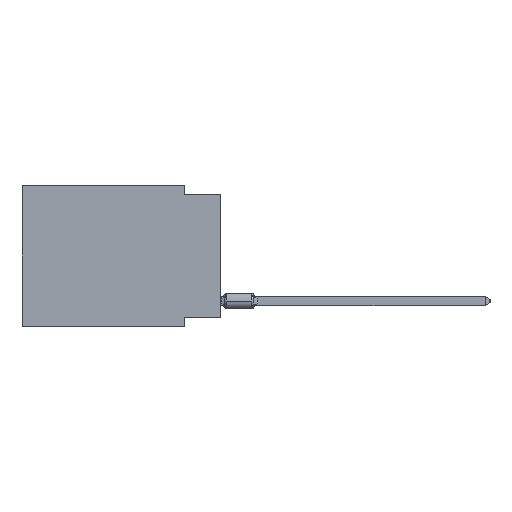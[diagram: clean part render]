
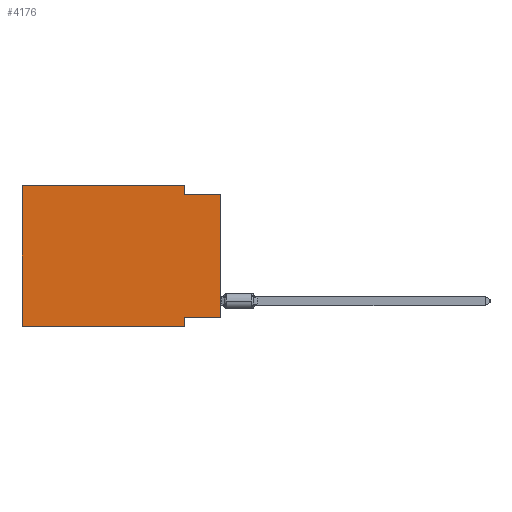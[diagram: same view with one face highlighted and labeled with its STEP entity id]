
A CAD part, left-side view. The second image highlights one B-rep face of the part: STEP entity #4176.
In plain terms, the highlighted planar face has unit normal (-1, 0, 0).
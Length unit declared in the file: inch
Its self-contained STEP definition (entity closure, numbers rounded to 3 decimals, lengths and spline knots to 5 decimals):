
#361 = AXIS2_PLACEMENT_3D ( 'NONE', #6484, #21641, #18497 ) ;
#648 = LINE ( 'NONE', #14672, #15984 ) ;
#899 = ORIENTED_EDGE ( 'NONE', *, *, #13666, .F. ) ;
#2309 = VERTEX_POINT ( 'NONE', #17022 ) ;
#2462 = VECTOR ( 'NONE', #12672, 39.37008 ) ;
#2760 = LINE ( 'NONE', #16469, #10200 ) ;
#2993 = CARTESIAN_POINT ( 'NONE',  ( 0., 0.55, -0.39 ) ) ;
#3290 = EDGE_CURVE ( 'NONE', #9342, #16589, #8246, .T. ) ;
#3692 = LINE ( 'NONE', #15807, #15555 ) ;
#3837 = VECTOR ( 'NONE', #22190, 39.37008 ) ;
#4170 = CARTESIAN_POINT ( 'NONE',  ( 0., 0.1, 0. ) ) ;
#4176 = ADVANCED_FACE ( 'NONE', ( #12927 ), #14635, .F. ) ;
#4563 = ORIENTED_EDGE ( 'NONE', *, *, #20878, .F. ) ;
#4985 = ORIENTED_EDGE ( 'NONE', *, *, #10043, .F. ) ;
#4989 = LINE ( 'NONE', #22304, #3837 ) ;
#6184 = EDGE_CURVE ( 'NONE', #16589, #2309, #3692, .T. ) ;
#6304 = EDGE_CURVE ( 'NONE', #8021, #17239, #14425, .T. ) ;
#6484 = CARTESIAN_POINT ( 'NONE',  ( 0., 0.55, 0. ) ) ;
#7195 = DIRECTION ( 'NONE',  ( 0., -1., 0. ) ) ;
#7353 = DIRECTION ( 'NONE',  ( 0., 0., -1. ) ) ;
#7598 = CARTESIAN_POINT ( 'NONE',  ( 0., 0., -0.025 ) ) ;
#7630 = CARTESIAN_POINT ( 'NONE',  ( 0., 0., 0. ) ) ;
#7696 = LINE ( 'NONE', #9282, #2462 ) ;
#8021 = VERTEX_POINT ( 'NONE', #22087 ) ;
#8033 = ORIENTED_EDGE ( 'NONE', *, *, #6304, .T. ) ;
#8160 = VECTOR ( 'NONE', #22046, 39.37008 ) ;
#8246 = LINE ( 'NONE', #9600, #8160 ) ;
#8385 = VECTOR ( 'NONE', #7353, 39.37008 ) ;
#8571 = CARTESIAN_POINT ( 'NONE',  ( 0., 0.1, -0.025 ) ) ;
#8937 = VERTEX_POINT ( 'NONE', #21914 ) ;
#9002 = DIRECTION ( 'NONE',  ( 0., 0., 1. ) ) ;
#9270 = LINE ( 'NONE', #4170, #8385 ) ;
#9282 = CARTESIAN_POINT ( 'NONE',  ( 0., 0.1, -0.39 ) ) ;
#9293 = EDGE_CURVE ( 'NONE', #13123, #17239, #2760, .T. ) ;
#9342 = VERTEX_POINT ( 'NONE', #2993 ) ;
#9600 = CARTESIAN_POINT ( 'NONE',  ( 0., 0.55, 0. ) ) ;
#9711 = EDGE_LOOP ( 'NONE', ( #8033, #14088, #4563, #15229, #11040, #15368, #899, #4985 ) ) ;
#10043 = EDGE_CURVE ( 'NONE', #8021, #15259, #648, .T. ) ;
#10200 = VECTOR ( 'NONE', #11245, 39.37008 ) ;
#10288 = CARTESIAN_POINT ( 'NONE',  ( 0., 0.55, 0. ) ) ;
#11040 = ORIENTED_EDGE ( 'NONE', *, *, #3290, .F. ) ;
#11245 = DIRECTION ( 'NONE',  ( 0., -1., 0. ) ) ;
#11375 = CARTESIAN_POINT ( 'NONE',  ( 0., 0.1, -0.365 ) ) ;
#12672 = DIRECTION ( 'NONE',  ( 0., 0., -1. ) ) ;
#12927 = FACE_OUTER_BOUND ( 'NONE', #9711, .T. ) ;
#13123 = VERTEX_POINT ( 'NONE', #8571 ) ;
#13666 = EDGE_CURVE ( 'NONE', #15259, #8937, #7696, .T. ) ;
#14088 = ORIENTED_EDGE ( 'NONE', *, *, #9293, .F. ) ;
#14425 = LINE ( 'NONE', #7630, #18825 ) ;
#14564 = DIRECTION ( 'NONE',  ( 0., 1., 0. ) ) ;
#14635 = PLANE ( 'NONE',  #361 ) ;
#14672 = CARTESIAN_POINT ( 'NONE',  ( 0., 0., -0.365 ) ) ;
#14995 = EDGE_CURVE ( 'NONE', #9342, #8937, #4989, .T. ) ;
#15229 = ORIENTED_EDGE ( 'NONE', *, *, #6184, .F. ) ;
#15259 = VERTEX_POINT ( 'NONE', #11375 ) ;
#15368 = ORIENTED_EDGE ( 'NONE', *, *, #14995, .T. ) ;
#15555 = VECTOR ( 'NONE', #7195, 39.37008 ) ;
#15807 = CARTESIAN_POINT ( 'NONE',  ( 0., 0.55, 0. ) ) ;
#15984 = VECTOR ( 'NONE', #14564, 39.37008 ) ;
#16469 = CARTESIAN_POINT ( 'NONE',  ( 0., 0., -0.025 ) ) ;
#16589 = VERTEX_POINT ( 'NONE', #10288 ) ;
#17022 = CARTESIAN_POINT ( 'NONE',  ( 0., 0.1, 0. ) ) ;
#17239 = VERTEX_POINT ( 'NONE', #7598 ) ;
#18497 = DIRECTION ( 'NONE',  ( 0., 0., -1. ) ) ;
#18825 = VECTOR ( 'NONE', #9002, 39.37008 ) ;
#20878 = EDGE_CURVE ( 'NONE', #2309, #13123, #9270, .T. ) ;
#21641 = DIRECTION ( 'NONE',  ( 1., 0., 0. ) ) ;
#21914 = CARTESIAN_POINT ( 'NONE',  ( 0., 0.1, -0.39 ) ) ;
#22046 = DIRECTION ( 'NONE',  ( 0., 0., 1. ) ) ;
#22087 = CARTESIAN_POINT ( 'NONE',  ( 0., 0., -0.365 ) ) ;
#22190 = DIRECTION ( 'NONE',  ( 0., -1., 0. ) ) ;
#22304 = CARTESIAN_POINT ( 'NONE',  ( 0., 0.55, -0.39 ) ) ;
